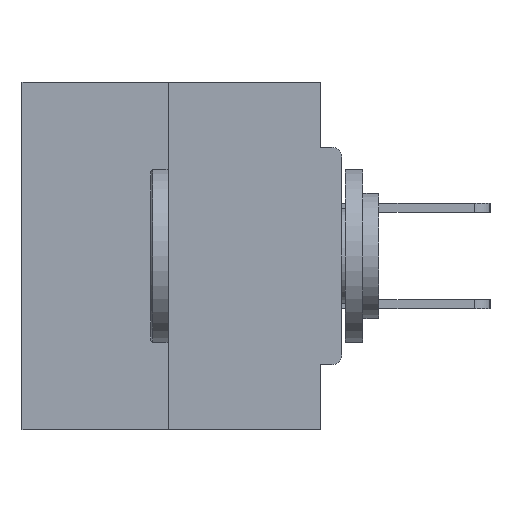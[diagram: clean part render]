
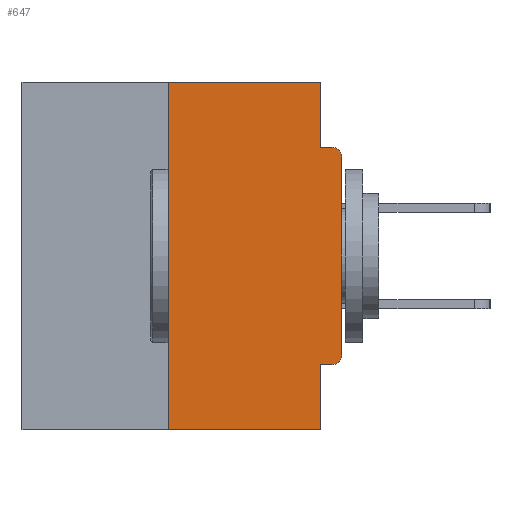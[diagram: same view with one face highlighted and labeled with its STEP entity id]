
A CAD part, left-side view. The second image highlights one B-rep face of the part: STEP entity #647.
In plain terms, the highlighted planar face has unit normal (-1, 0, 0).
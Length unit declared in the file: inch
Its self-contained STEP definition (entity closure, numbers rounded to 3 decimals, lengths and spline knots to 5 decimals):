
#315 = LINE ( 'NONE', #10608, #19025 ) ;
#339 = VERTEX_POINT ( 'NONE', #29968 ) ;
#647 = ADVANCED_FACE ( 'NONE', ( #12593 ), #22900, .F. ) ;
#709 = AXIS2_PLACEMENT_3D ( 'NONE', #14612, #32369, #8927 ) ;
#1105 = VERTEX_POINT ( 'NONE', #36493 ) ;
#1154 = VECTOR ( 'NONE', #17818, 39.37008 ) ;
#1210 = EDGE_CURVE ( 'NONE', #19693, #26789, #20755, .T. ) ;
#1253 = LINE ( 'NONE', #2430, #31324 ) ;
#2414 = ORIENTED_EDGE ( 'NONE', *, *, #20836, .F. ) ;
#2430 = CARTESIAN_POINT ( 'NONE',  ( 0., 0.25, 0. ) ) ;
#2645 = DIRECTION ( 'NONE',  ( 0., 0., -1. ) ) ;
#3306 = CARTESIAN_POINT ( 'NONE',  ( 0., 0.46, 0. ) ) ;
#5101 = CARTESIAN_POINT ( 'NONE',  ( 0., 0., -0.4065 ) ) ;
#6366 = EDGE_CURVE ( 'NONE', #34486, #27930, #23593, .T. ) ;
#6534 = DIRECTION ( 'NONE',  ( 0., 0., -1. ) ) ;
#6819 = VERTEX_POINT ( 'NONE', #11530 ) ;
#7065 = ORIENTED_EDGE ( 'NONE', *, *, #10789, .T. ) ;
#7155 = AXIS2_PLACEMENT_3D ( 'NONE', #34584, #28723, #22728 ) ;
#7866 = CARTESIAN_POINT ( 'NONE',  ( 0., 0.031, 0. ) ) ;
#8602 = CARTESIAN_POINT ( 'NONE',  ( 0., 0.25, 0. ) ) ;
#8927 = DIRECTION ( 'NONE',  ( 0., 0., -1. ) ) ;
#8959 = ORIENTED_EDGE ( 'NONE', *, *, #20191, .F. ) ;
#9127 = VECTOR ( 'NONE', #17718, 39.37008 ) ;
#9608 = LINE ( 'NONE', #37164, #22326 ) ;
#9942 = VECTOR ( 'NONE', #6534, 39.37008 ) ;
#10045 = DIRECTION ( 'NONE',  ( 0., 0., 1. ) ) ;
#10608 = CARTESIAN_POINT ( 'NONE',  ( 0., 0., -0.0935 ) ) ;
#10789 = EDGE_CURVE ( 'NONE', #1105, #34486, #9608, .T. ) ;
#11530 = CARTESIAN_POINT ( 'NONE',  ( 0., 0.031, -0.4065 ) ) ;
#12593 = FACE_OUTER_BOUND ( 'NONE', #24315, .T. ) ;
#13632 = VECTOR ( 'NONE', #31417, 39.37008 ) ;
#13881 = DIRECTION ( 'NONE',  ( 0., -1., 0. ) ) ;
#14612 = CARTESIAN_POINT ( 'NONE',  ( 0., 0.015, -0.3915 ) ) ;
#14860 = CARTESIAN_POINT ( 'NONE',  ( 0., 0.031, -0.5 ) ) ;
#14882 = CARTESIAN_POINT ( 'NONE',  ( 0., 0.031, 0. ) ) ;
#15030 = VERTEX_POINT ( 'NONE', #8602 ) ;
#15405 = CARTESIAN_POINT ( 'NONE',  ( 0., 0.031, -0.0935 ) ) ;
#15518 = ORIENTED_EDGE ( 'NONE', *, *, #1210, .T. ) ;
#17500 = EDGE_CURVE ( 'NONE', #33190, #27930, #315, .T. ) ;
#17710 = AXIS2_PLACEMENT_3D ( 'NONE', #28650, #34637, #2645 ) ;
#17718 = DIRECTION ( 'NONE',  ( 0., -1., 0. ) ) ;
#17818 = DIRECTION ( 'NONE',  ( 0., -1., 0. ) ) ;
#18281 = ORIENTED_EDGE ( 'NONE', *, *, #17500, .F. ) ;
#19025 = VECTOR ( 'NONE', #13881, 39.37008 ) ;
#19124 = ORIENTED_EDGE ( 'NONE', *, *, #6366, .T. ) ;
#19693 = VERTEX_POINT ( 'NONE', #36629 ) ;
#20191 = EDGE_CURVE ( 'NONE', #6819, #26789, #31317, .T. ) ;
#20351 = CARTESIAN_POINT ( 'NONE',  ( 0., 0.46, -0.5 ) ) ;
#20498 = LINE ( 'NONE', #7866, #13632 ) ;
#20755 = LINE ( 'NONE', #20351, #1154 ) ;
#20836 = EDGE_CURVE ( 'NONE', #19693, #15030, #1253, .T. ) ;
#22326 = VECTOR ( 'NONE', #10045, 39.37008 ) ;
#22728 = DIRECTION ( 'NONE',  ( 0., 0., -1. ) ) ;
#22900 = PLANE ( 'NONE',  #17710 ) ;
#23593 = CIRCLE ( 'NONE', #7155, 0.015 ) ;
#23677 = LINE ( 'NONE', #3306, #9127 ) ;
#24315 = EDGE_LOOP ( 'NONE', ( #26169, #2414, #15518, #8959, #37174, #25017, #7065, #19124, #18281, #27533 ) ) ;
#25017 = ORIENTED_EDGE ( 'NONE', *, *, #37365, .T. ) ;
#25829 = DIRECTION ( 'NONE',  ( 0., 1., 0. ) ) ;
#26169 = ORIENTED_EDGE ( 'NONE', *, *, #29842, .F. ) ;
#26522 = CARTESIAN_POINT ( 'NONE',  ( 0., 0.031, -0.5 ) ) ;
#26744 = CARTESIAN_POINT ( 'NONE',  ( 0., 0.015, -0.0935 ) ) ;
#26789 = VERTEX_POINT ( 'NONE', #14860 ) ;
#27533 = ORIENTED_EDGE ( 'NONE', *, *, #30064, .F. ) ;
#27930 = VERTEX_POINT ( 'NONE', #26744 ) ;
#28115 = VECTOR ( 'NONE', #25829, 39.37008 ) ;
#28650 = CARTESIAN_POINT ( 'NONE',  ( 0., 0.46, 0. ) ) ;
#28723 = DIRECTION ( 'NONE',  ( -1., 0., 0. ) ) ;
#29220 = VERTEX_POINT ( 'NONE', #14882 ) ;
#29842 = EDGE_CURVE ( 'NONE', #15030, #29220, #23677, .T. ) ;
#29968 = CARTESIAN_POINT ( 'NONE',  ( 0., 0.015, -0.4065 ) ) ;
#30053 = CIRCLE ( 'NONE', #709, 0.015 ) ;
#30064 = EDGE_CURVE ( 'NONE', #29220, #33190, #20498, .T. ) ;
#31317 = LINE ( 'NONE', #26522, #9942 ) ;
#31324 = VECTOR ( 'NONE', #34052, 39.37008 ) ;
#31417 = DIRECTION ( 'NONE',  ( 0., 0., -1. ) ) ;
#31572 = CARTESIAN_POINT ( 'NONE',  ( 0., 0., -0.1085 ) ) ;
#32369 = DIRECTION ( 'NONE',  ( -1., 0., 0. ) ) ;
#33190 = VERTEX_POINT ( 'NONE', #15405 ) ;
#34052 = DIRECTION ( 'NONE',  ( 0., 0., 1. ) ) ;
#34486 = VERTEX_POINT ( 'NONE', #31572 ) ;
#34551 = EDGE_CURVE ( 'NONE', #339, #6819, #34952, .T. ) ;
#34584 = CARTESIAN_POINT ( 'NONE',  ( 0., 0.015, -0.1085 ) ) ;
#34637 = DIRECTION ( 'NONE',  ( 1., 0., 0. ) ) ;
#34952 = LINE ( 'NONE', #5101, #28115 ) ;
#36493 = CARTESIAN_POINT ( 'NONE',  ( 0., 0., -0.3915 ) ) ;
#36629 = CARTESIAN_POINT ( 'NONE',  ( 0., 0.25, -0.5 ) ) ;
#37164 = CARTESIAN_POINT ( 'NONE',  ( 0., 0., 0. ) ) ;
#37174 = ORIENTED_EDGE ( 'NONE', *, *, #34551, .F. ) ;
#37365 = EDGE_CURVE ( 'NONE', #339, #1105, #30053, .T. ) ;
